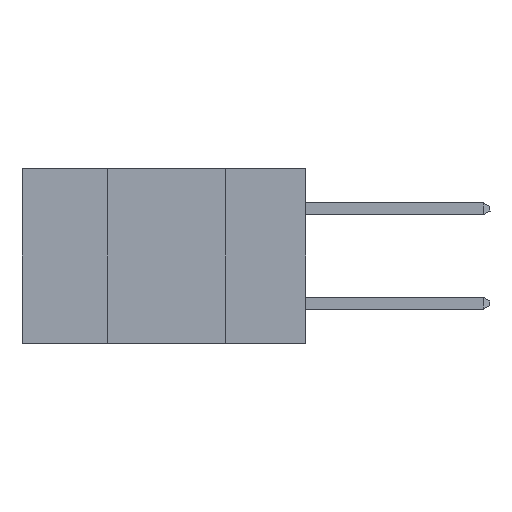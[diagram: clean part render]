
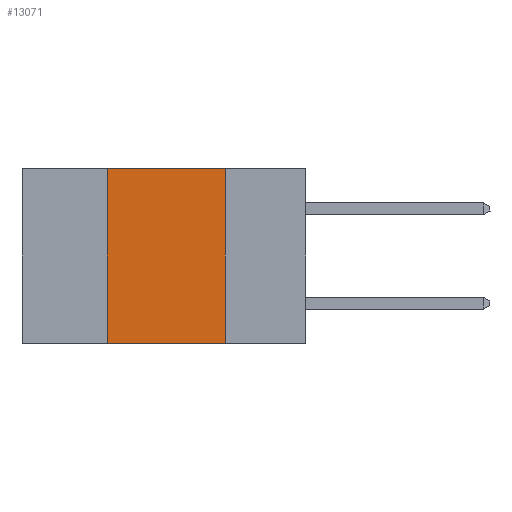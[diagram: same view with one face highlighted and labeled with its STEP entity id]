
A CAD part, left-side view. The second image highlights one B-rep face of the part: STEP entity #13071.
In plain terms, the highlighted planar face has unit normal (-1, 0, 0).
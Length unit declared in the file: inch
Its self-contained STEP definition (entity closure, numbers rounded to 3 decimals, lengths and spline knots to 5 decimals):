
#289 = LINE ( 'NONE', #8326, #7148 ) ;
#1224 = EDGE_CURVE ( 'NONE', #6560, #3447, #14410, .T. ) ;
#1318 = CARTESIAN_POINT ( 'NONE',  ( 0., 0.17, -0.37 ) ) ;
#1735 = DIRECTION ( 'NONE',  ( 0., 0., -1. ) ) ;
#2241 = CARTESIAN_POINT ( 'NONE',  ( 0., 0.42, 0. ) ) ;
#3262 = VERTEX_POINT ( 'NONE', #1318 ) ;
#3369 = VECTOR ( 'NONE', #15659, 39.37008 ) ;
#3447 = VERTEX_POINT ( 'NONE', #2241 ) ;
#3450 = CARTESIAN_POINT ( 'NONE',  ( 0., 0.6, 0. ) ) ;
#3553 = DIRECTION ( 'NONE',  ( 1., 0., 0. ) ) ;
#4219 = ORIENTED_EDGE ( 'NONE', *, *, #16477, .T. ) ;
#4635 = VECTOR ( 'NONE', #14938, 39.37008 ) ;
#6560 = VERTEX_POINT ( 'NONE', #21374 ) ;
#7148 = VECTOR ( 'NONE', #1735, 39.37008 ) ;
#7257 = CARTESIAN_POINT ( 'NONE',  ( 0., 0.42, 0. ) ) ;
#7415 = CARTESIAN_POINT ( 'NONE',  ( 0., 0.17, 0. ) ) ;
#8326 = CARTESIAN_POINT ( 'NONE',  ( 0., 0.17, 0. ) ) ;
#8362 = CARTESIAN_POINT ( 'NONE',  ( 0., 0.6, -0.37 ) ) ;
#12032 = EDGE_LOOP ( 'NONE', ( #19518, #18744, #12337, #4219 ) ) ;
#12337 = ORIENTED_EDGE ( 'NONE', *, *, #1224, .F. ) ;
#12479 = EDGE_CURVE ( 'NONE', #14692, #3262, #289, .T. ) ;
#13071 = ADVANCED_FACE ( 'NONE', ( #14983 ), #13629, .F. ) ;
#13629 = PLANE ( 'NONE',  #20315 ) ;
#14410 = LINE ( 'NONE', #7257, #3369 ) ;
#14692 = VERTEX_POINT ( 'NONE', #7415 ) ;
#14875 = LINE ( 'NONE', #3450, #21157 ) ;
#14938 = DIRECTION ( 'NONE',  ( 0., -1., 0. ) ) ;
#14983 = FACE_OUTER_BOUND ( 'NONE', #12032, .T. ) ;
#15131 = DIRECTION ( 'NONE',  ( 0., -1., 0. ) ) ;
#15659 = DIRECTION ( 'NONE',  ( 0., 0., 1. ) ) ;
#16342 = DIRECTION ( 'NONE',  ( 0., 0., -1. ) ) ;
#16477 = EDGE_CURVE ( 'NONE', #6560, #3262, #18549, .T. ) ;
#17082 = EDGE_CURVE ( 'NONE', #3447, #14692, #14875, .T. ) ;
#18549 = LINE ( 'NONE', #8362, #4635 ) ;
#18744 = ORIENTED_EDGE ( 'NONE', *, *, #17082, .F. ) ;
#19518 = ORIENTED_EDGE ( 'NONE', *, *, #12479, .F. ) ;
#19766 = CARTESIAN_POINT ( 'NONE',  ( 0., 0.6, 0. ) ) ;
#20315 = AXIS2_PLACEMENT_3D ( 'NONE', #19766, #3553, #16342 ) ;
#21157 = VECTOR ( 'NONE', #15131, 39.37008 ) ;
#21374 = CARTESIAN_POINT ( 'NONE',  ( 0., 0.42, -0.37 ) ) ;
